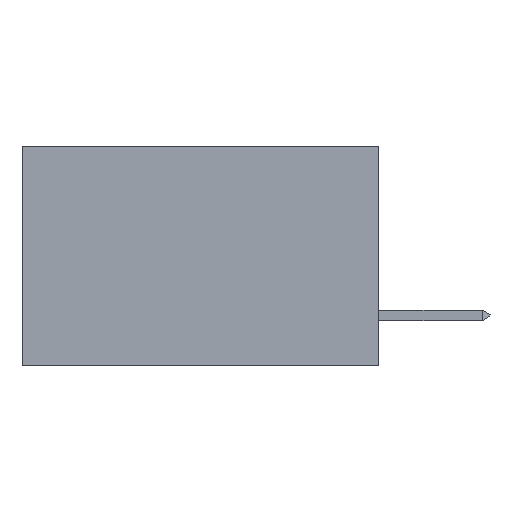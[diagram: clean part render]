
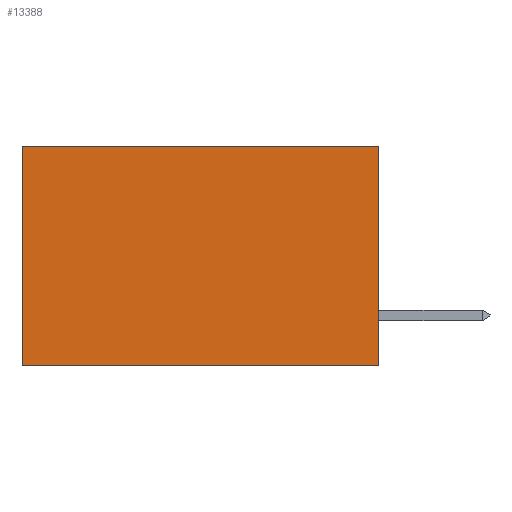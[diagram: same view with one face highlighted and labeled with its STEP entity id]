
A CAD part, left-side view. The second image highlights one B-rep face of the part: STEP entity #13388.
In plain terms, the highlighted planar face has unit normal (-1, 0, 0).
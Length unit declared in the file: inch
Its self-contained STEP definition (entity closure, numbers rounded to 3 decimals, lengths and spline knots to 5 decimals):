
#132 = CARTESIAN_POINT ( 'NONE',  ( 0.298, 0.6, 0. ) ) ;
#617 = ORIENTED_EDGE ( 'NONE', *, *, #2497, .F. ) ;
#896 = VECTOR ( 'NONE', #2192, 39.37008 ) ;
#2192 = DIRECTION ( 'NONE',  ( 0., 1., 0. ) ) ;
#2259 = DIRECTION ( 'NONE',  ( 0., 1., 0. ) ) ;
#2376 = EDGE_CURVE ( 'NONE', #12350, #25713, #2449, .T. ) ;
#2449 = LINE ( 'NONE', #17315, #20437 ) ;
#2497 = EDGE_CURVE ( 'NONE', #25713, #20600, #4980, .T. ) ;
#3443 = CARTESIAN_POINT ( 'NONE',  ( 0.298, 0., 0. ) ) ;
#4113 = CARTESIAN_POINT ( 'NONE',  ( 0.298, 0., -0.37 ) ) ;
#4445 = CARTESIAN_POINT ( 'NONE',  ( 0.298, 0.6, 0. ) ) ;
#4980 = LINE ( 'NONE', #24529, #21398 ) ;
#5169 = DIRECTION ( 'NONE',  ( 0., 0., -1. ) ) ;
#6247 = CARTESIAN_POINT ( 'NONE',  ( 0.298, 0., 0. ) ) ;
#7058 = DIRECTION ( 'NONE',  ( 0., 0., -1. ) ) ;
#7165 = LINE ( 'NONE', #6247, #896 ) ;
#8836 = DIRECTION ( 'NONE',  ( 1., 0., 0. ) ) ;
#9012 = PLANE ( 'NONE',  #21945 ) ;
#11043 = ORIENTED_EDGE ( 'NONE', *, *, #26144, .T. ) ;
#12350 = VERTEX_POINT ( 'NONE', #3443 ) ;
#12901 = DIRECTION ( 'NONE',  ( 0., 0., -1. ) ) ;
#13388 = ADVANCED_FACE ( 'NONE', ( #18256 ), #9012, .F. ) ;
#13960 = ORIENTED_EDGE ( 'NONE', *, *, #17188, .T. ) ;
#14687 = ORIENTED_EDGE ( 'NONE', *, *, #2376, .F. ) ;
#16937 = EDGE_LOOP ( 'NONE', ( #13960, #617, #14687, #11043 ) ) ;
#17122 = CARTESIAN_POINT ( 'NONE',  ( 0.298, 0., 0. ) ) ;
#17188 = EDGE_CURVE ( 'NONE', #17521, #20600, #24641, .T. ) ;
#17315 = CARTESIAN_POINT ( 'NONE',  ( 0.298, 0., 0. ) ) ;
#17521 = VERTEX_POINT ( 'NONE', #132 ) ;
#18256 = FACE_OUTER_BOUND ( 'NONE', #16937, .T. ) ;
#18685 = CARTESIAN_POINT ( 'NONE',  ( 0.298, 0.6, -0.37 ) ) ;
#19239 = VECTOR ( 'NONE', #7058, 39.37008 ) ;
#20437 = VECTOR ( 'NONE', #5169, 39.37008 ) ;
#20600 = VERTEX_POINT ( 'NONE', #18685 ) ;
#21398 = VECTOR ( 'NONE', #2259, 39.37008 ) ;
#21945 = AXIS2_PLACEMENT_3D ( 'NONE', #17122, #8836, #12901 ) ;
#24529 = CARTESIAN_POINT ( 'NONE',  ( 0.298, 0., -0.37 ) ) ;
#24641 = LINE ( 'NONE', #4445, #19239 ) ;
#25713 = VERTEX_POINT ( 'NONE', #4113 ) ;
#26144 = EDGE_CURVE ( 'NONE', #12350, #17521, #7165, .T. ) ;
